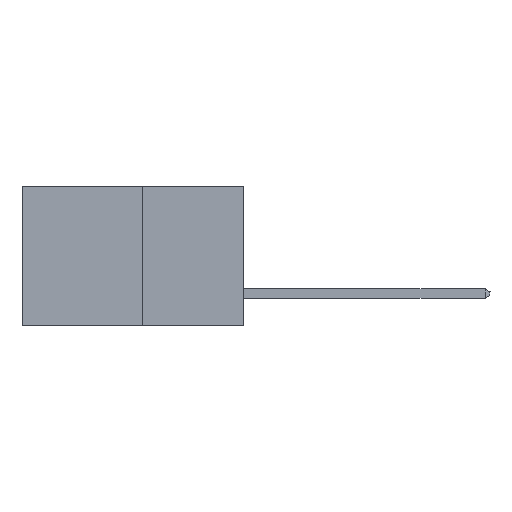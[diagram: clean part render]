
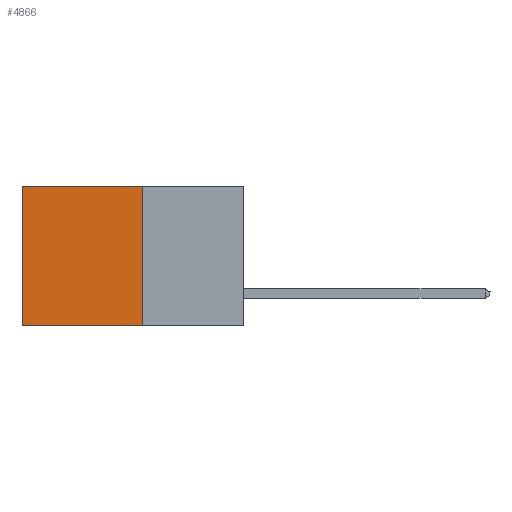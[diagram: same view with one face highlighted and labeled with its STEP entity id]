
A CAD part, left-side view. The second image highlights one B-rep face of the part: STEP entity #4866.
In plain terms, the highlighted planar face has unit normal (-1, 0, 0).
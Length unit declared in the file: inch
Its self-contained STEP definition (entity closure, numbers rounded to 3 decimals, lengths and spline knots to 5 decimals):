
#19 = DIRECTION ( 'NONE',  ( 1., 0., 0. ) ) ;
#103 = PLANE ( 'NONE',  #5505 ) ;
#842 = CARTESIAN_POINT ( 'NONE',  ( 0.277, 0.59, 0. ) ) ;
#863 = DIRECTION ( 'NONE',  ( 0., 0., -1. ) ) ;
#1004 = VECTOR ( 'NONE', #5364, 39.37008 ) ;
#1069 = EDGE_CURVE ( 'NONE', #13364, #10392, #10743, .T. ) ;
#1173 = VECTOR ( 'NONE', #863, 39.37008 ) ;
#1791 = CARTESIAN_POINT ( 'NONE',  ( 0.277, 0.59, -0.37 ) ) ;
#1874 = VERTEX_POINT ( 'NONE', #842 ) ;
#2853 = FACE_OUTER_BOUND ( 'NONE', #9230, .T. ) ;
#3311 = CARTESIAN_POINT ( 'NONE',  ( 0.277, 0.27, -0.37 ) ) ;
#4437 = ORIENTED_EDGE ( 'NONE', *, *, #13874, .T. ) ;
#4866 = ADVANCED_FACE ( 'NONE', ( #2853 ), #103, .F. ) ;
#5364 = DIRECTION ( 'NONE',  ( 0., 1., 0. ) ) ;
#5394 = CARTESIAN_POINT ( 'NONE',  ( 0.277, 0.27, -0.37 ) ) ;
#5481 = ORIENTED_EDGE ( 'NONE', *, *, #5892, .T. ) ;
#5505 = AXIS2_PLACEMENT_3D ( 'NONE', #13760, #19, #9153 ) ;
#5892 = EDGE_CURVE ( 'NONE', #6558, #1874, #7028, .T. ) ;
#6178 = CARTESIAN_POINT ( 'NONE',  ( 0.277, 0.27, 0. ) ) ;
#6558 = VERTEX_POINT ( 'NONE', #12290 ) ;
#7028 = LINE ( 'NONE', #6178, #1004 ) ;
#7786 = ORIENTED_EDGE ( 'NONE', *, *, #1069, .F. ) ;
#7869 = VECTOR ( 'NONE', #13717, 39.37008 ) ;
#8126 = ORIENTED_EDGE ( 'NONE', *, *, #9456, .F. ) ;
#9153 = DIRECTION ( 'NONE',  ( 0., 0., -1. ) ) ;
#9192 = LINE ( 'NONE', #11868, #11691 ) ;
#9230 = EDGE_LOOP ( 'NONE', ( #4437, #7786, #8126, #5481 ) ) ;
#9456 = EDGE_CURVE ( 'NONE', #6558, #13364, #13196, .T. ) ;
#10392 = VERTEX_POINT ( 'NONE', #1791 ) ;
#10743 = LINE ( 'NONE', #3311, #7869 ) ;
#11691 = VECTOR ( 'NONE', #13766, 39.37008 ) ;
#11868 = CARTESIAN_POINT ( 'NONE',  ( 0.277, 0.59, -0.37 ) ) ;
#12290 = CARTESIAN_POINT ( 'NONE',  ( 0.277, 0.27, 0. ) ) ;
#13196 = LINE ( 'NONE', #13925, #1173 ) ;
#13364 = VERTEX_POINT ( 'NONE', #5394 ) ;
#13717 = DIRECTION ( 'NONE',  ( 0., 1., 0. ) ) ;
#13760 = CARTESIAN_POINT ( 'NONE',  ( 0.277, 0.27, -0.37 ) ) ;
#13766 = DIRECTION ( 'NONE',  ( 0., 0., -1. ) ) ;
#13874 = EDGE_CURVE ( 'NONE', #1874, #10392, #9192, .T. ) ;
#13925 = CARTESIAN_POINT ( 'NONE',  ( 0.277, 0.27, -0.37 ) ) ;
